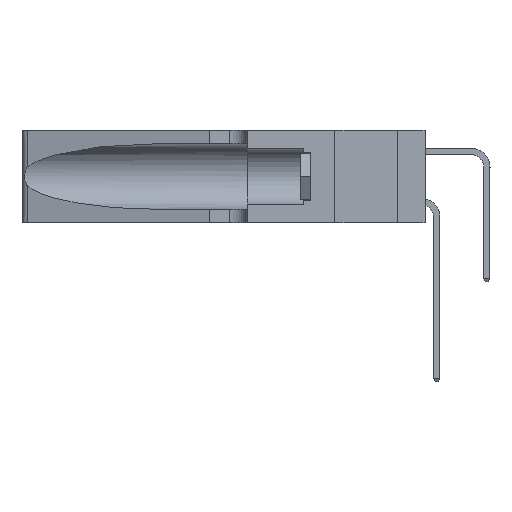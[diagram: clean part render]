
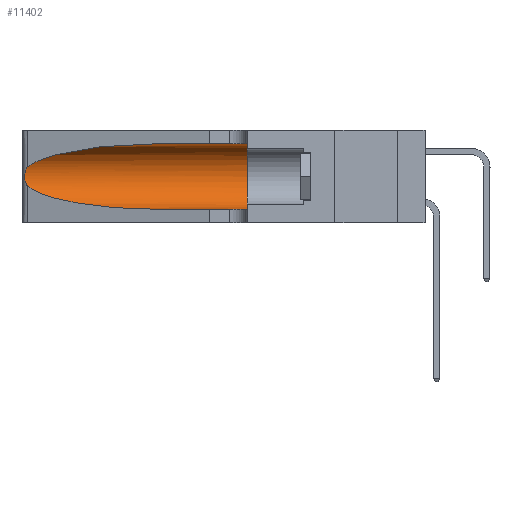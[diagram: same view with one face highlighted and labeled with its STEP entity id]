
A CAD part, left-side view. The second image highlights one B-rep face of the part: STEP entity #11402.
In plain terms, the highlighted cylindrical face has radius 3.308 mm (diameter 6.617 mm), a partial arc.
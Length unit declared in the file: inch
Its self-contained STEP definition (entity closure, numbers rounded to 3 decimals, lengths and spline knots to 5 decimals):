
#1039 = VECTOR ( 'NONE', #18615, 39.37008 ) ;
#1160 = CARTESIAN_POINT ( 'NONE',  ( 0.25856, 1.23593, 0.16098 ) ) ;
#1310 = B_SPLINE_CURVE_WITH_KNOTS ( 'NONE', 3,
 ( #26703, #29935, #10735, #33144, #13972, #36345, #17215, #39535, #20423, #1160, #23637, #4401, #26846, #7629 ),
 .UNSPECIFIED., .F., .F.,
 ( 4, 2, 2, 2, 2, 2, 4 ),
 ( 0., 0.00027, 0.00053, 0.00107, 0.0016, 0.00187, 0.00214 ),
 .UNSPECIFIED. ) ;
#1555 =( BOUNDED_CURVE ( )  B_SPLINE_CURVE ( 3, ( #21958, #2701, #5909, #28372 ),
 .UNSPECIFIED., .F., .T. ) 
 B_SPLINE_CURVE_WITH_KNOTS ( ( 4, 4 ),
 ( 1.5708, 2.84003 ),
 .UNSPECIFIED. ) 
 CURVE ( )  GEOMETRIC_REPRESENTATION_ITEM ( )  RATIONAL_B_SPLINE_CURVE ( ( 1., 0.87, 0.87, 1. ) ) 
 REPRESENTATION_ITEM ( '' )  );
#2295 = VERTEX_POINT ( 'NONE', #33315 ) ;
#2520 = VERTEX_POINT ( 'NONE', #37604 ) ;
#2701 = CARTESIAN_POINT ( 'NONE',  ( 0.18966, 0.96281, 0.31525 ) ) ;
#3087 = DIRECTION ( 'NONE',  ( 0., 0., -1. ) ) ;
#4081 = CARTESIAN_POINT ( 'NONE',  ( 0.1305, 0.72297, 0.05475 ) ) ;
#4401 = CARTESIAN_POINT ( 'NONE',  ( 0.25639, 1.23186, 0.15144 ) ) ;
#4923 = CARTESIAN_POINT ( 'NONE',  ( 0.1305, 0.35, 0.31525 ) ) ;
#5909 = CARTESIAN_POINT ( 'NONE',  ( 0.2373, 1.15595, 0.28018 ) ) ;
#6230 = ORIENTED_EDGE ( 'NONE', *, *, #16533, .F. ) ;
#7337 = VERTEX_POINT ( 'NONE', #4923 ) ;
#7629 = CARTESIAN_POINT ( 'NONE',  ( 0.25487, 1.22718, 0.14631 ) ) ;
#8191 = DIRECTION ( 'NONE',  ( 0., 1., 0. ) ) ;
#9068 = CARTESIAN_POINT ( 'NONE',  ( 0.1305, 1.61858, 0.31525 ) ) ;
#9467 = ORIENTED_EDGE ( 'NONE', *, *, #28981, .T. ) ;
#10735 = CARTESIAN_POINT ( 'NONE',  ( 0.25639, 1.23184, 0.21858 ) ) ;
#10915 = ORIENTED_EDGE ( 'NONE', *, *, #36061, .T. ) ;
#11402 = ADVANCED_FACE ( 'NONE', ( #41208 ), #31745, .F. ) ;
#12164 = CARTESIAN_POINT ( 'NONE',  ( 0.25487, 1.22718, 0.14631 ) ) ;
#12654 = CARTESIAN_POINT ( 'NONE',  ( 0.1305, 1.61858, 0.185 ) ) ;
#13972 = CARTESIAN_POINT ( 'NONE',  ( 0.25854, 1.2359, 0.20912 ) ) ;
#15396 = CARTESIAN_POINT ( 'NONE',  ( 0.1305, 0.72297, 0.05475 ) ) ;
#15831 = EDGE_LOOP ( 'NONE', ( #10915, #9467, #34349, #31053, #6230, #32332 ) ) ;
#16100 = VERTEX_POINT ( 'NONE', #4081 ) ;
#16533 = EDGE_CURVE ( 'NONE', #7337, #2295, #28691, .T. ) ;
#17215 = CARTESIAN_POINT ( 'NONE',  ( 0.26075, 1.23896, 0.19203 ) ) ;
#18147 = LINE ( 'NONE', #9068, #1039 ) ;
#18615 = DIRECTION ( 'NONE',  ( 0., -1., 0. ) ) ;
#19131 = DIRECTION ( 'NONE',  ( 0., -1., 0. ) ) ;
#20423 = CARTESIAN_POINT ( 'NONE',  ( 0.26017, 1.23833, 0.17102 ) ) ;
#21958 = CARTESIAN_POINT ( 'NONE',  ( 0.1305, 0.72297, 0.31525 ) ) ;
#22901 =( BOUNDED_CURVE ( )  B_SPLINE_CURVE ( 3, ( #12164, #31360, #34544, #15396 ),
 .UNSPECIFIED., .F., .T. ) 
 B_SPLINE_CURVE_WITH_KNOTS ( ( 4, 4 ),
 ( 3.44316, 4.71239 ),
 .UNSPECIFIED. ) 
 CURVE ( )  GEOMETRIC_REPRESENTATION_ITEM ( )  RATIONAL_B_SPLINE_CURVE ( ( 1., 0.87, 0.87, 1. ) ) 
 REPRESENTATION_ITEM ( '' )  );
#23637 = CARTESIAN_POINT ( 'NONE',  ( 0.25789, 1.23486, 0.15765 ) ) ;
#24163 = CARTESIAN_POINT ( 'NONE',  ( 0.1305, 0.72297, 0.31525 ) ) ;
#24433 = CARTESIAN_POINT ( 'NONE',  ( 0.1305, 1.61858, 0.05475 ) ) ;
#26703 = CARTESIAN_POINT ( 'NONE',  ( 0.25487, 1.22718, 0.22369 ) ) ;
#26846 = CARTESIAN_POINT ( 'NONE',  ( 0.25555, 1.22993, 0.14849 ) ) ;
#27406 = CARTESIAN_POINT ( 'NONE',  ( 0.1305, 0.35, 0.185 ) ) ;
#27648 = DIRECTION ( 'NONE',  ( 0., -1., 0. ) ) ;
#28242 = CARTESIAN_POINT ( 'NONE',  ( 0.25487, 1.22718, 0.14631 ) ) ;
#28372 = CARTESIAN_POINT ( 'NONE',  ( 0.25487, 1.22718, 0.22369 ) ) ;
#28691 = CIRCLE ( 'NONE', #39412, 0.13025 ) ;
#28981 = EDGE_CURVE ( 'NONE', #2520, #39229, #1310, .T. ) ;
#29935 = CARTESIAN_POINT ( 'NONE',  ( 0.25555, 1.22994, 0.2215 ) ) ;
#30073 = VECTOR ( 'NONE', #27648, 39.37008 ) ;
#30630 = DIRECTION ( 'NONE',  ( 0., 0., 1. ) ) ;
#31053 = ORIENTED_EDGE ( 'NONE', *, *, #39767, .T. ) ;
#31091 = EDGE_CURVE ( 'NONE', #31611, #7337, #18147, .T. ) ;
#31360 = CARTESIAN_POINT ( 'NONE',  ( 0.2373, 1.15595, 0.08982 ) ) ;
#31611 = VERTEX_POINT ( 'NONE', #24163 ) ;
#31745 = CYLINDRICAL_SURFACE ( 'NONE', #38502, 0.13025 ) ;
#32332 = ORIENTED_EDGE ( 'NONE', *, *, #31091, .F. ) ;
#33144 = CARTESIAN_POINT ( 'NONE',  ( 0.25787, 1.23484, 0.2124 ) ) ;
#33315 = CARTESIAN_POINT ( 'NONE',  ( 0.1305, 0.35, 0.05475 ) ) ;
#34349 = ORIENTED_EDGE ( 'NONE', *, *, #37389, .T. ) ;
#34544 = CARTESIAN_POINT ( 'NONE',  ( 0.18966, 0.96281, 0.05475 ) ) ;
#36061 = EDGE_CURVE ( 'NONE', #31611, #2520, #1555, .T. ) ;
#36345 = CARTESIAN_POINT ( 'NONE',  ( 0.26018, 1.23835, 0.19895 ) ) ;
#37389 = EDGE_CURVE ( 'NONE', #39229, #16100, #22901, .T. ) ;
#37604 = CARTESIAN_POINT ( 'NONE',  ( 0.25487, 1.22718, 0.22369 ) ) ;
#38502 = AXIS2_PLACEMENT_3D ( 'NONE', #12654, #19131, #3087 ) ;
#38533 = LINE ( 'NONE', #24433, #30073 ) ;
#39229 = VERTEX_POINT ( 'NONE', #28242 ) ;
#39412 = AXIS2_PLACEMENT_3D ( 'NONE', #27406, #8191, #30630 ) ;
#39535 = CARTESIAN_POINT ( 'NONE',  ( 0.26075, 1.23896, 0.178 ) ) ;
#39767 = EDGE_CURVE ( 'NONE', #16100, #2295, #38533, .T. ) ;
#41208 = FACE_OUTER_BOUND ( 'NONE', #15831, .T. ) ;
